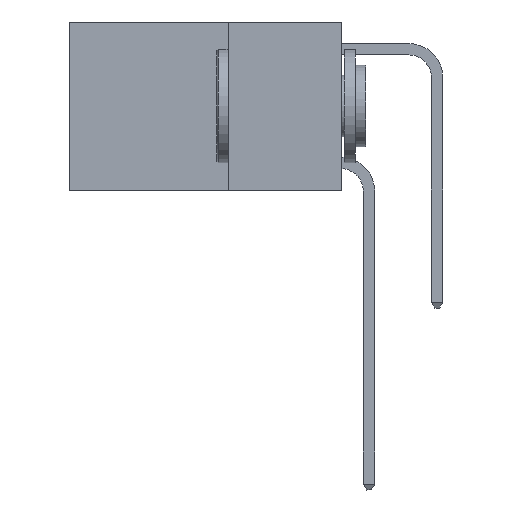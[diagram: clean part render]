
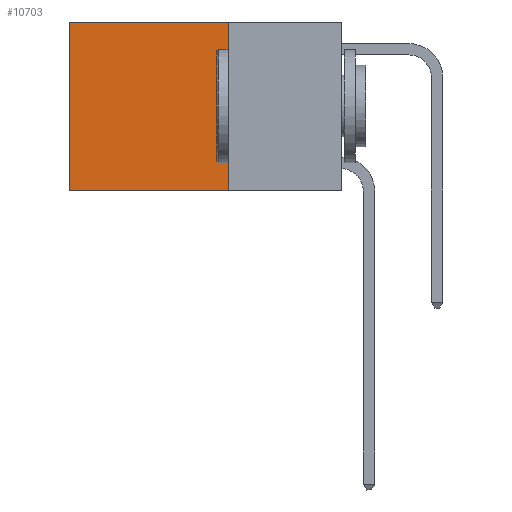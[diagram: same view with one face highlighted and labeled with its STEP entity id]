
A CAD part, left-side view. The second image highlights one B-rep face of the part: STEP entity #10703.
In plain terms, the highlighted planar face has unit normal (-1, 0, 0).
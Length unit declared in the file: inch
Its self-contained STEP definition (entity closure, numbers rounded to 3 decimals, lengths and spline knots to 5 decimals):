
#4 = CARTESIAN_POINT ( 'NONE',  ( 0.2625, 0.6, -0.37 ) ) ;
#459 = DIRECTION ( 'NONE',  ( 0., 0., -1. ) ) ;
#621 = VERTEX_POINT ( 'NONE', #10301 ) ;
#945 = VERTEX_POINT ( 'NONE', #8903 ) ;
#1092 = CARTESIAN_POINT ( 'NONE',  ( 0.2625, 0.6, 0. ) ) ;
#2034 = DIRECTION ( 'NONE',  ( 0., 0., -1. ) ) ;
#2357 = VECTOR ( 'NONE', #9716, 39.37008 ) ;
#2631 = EDGE_LOOP ( 'NONE', ( #8540, #8616, #8750, #8763 ) ) ;
#2666 = DIRECTION ( 'NONE',  ( 1., 0., 0. ) ) ;
#2970 = LINE ( 'NONE', #1092, #4953 ) ;
#3704 = EDGE_CURVE ( 'NONE', #621, #945, #8462, .T. ) ;
#3901 = VECTOR ( 'NONE', #4842, 39.37008 ) ;
#3992 = CARTESIAN_POINT ( 'NONE',  ( 0.2625, 0.25, -0.37 ) ) ;
#4842 = DIRECTION ( 'NONE',  ( 0., 1., 0. ) ) ;
#4857 = VERTEX_POINT ( 'NONE', #4 ) ;
#4953 = VECTOR ( 'NONE', #2034, 39.37008 ) ;
#5801 = LINE ( 'NONE', #3992, #3901 ) ;
#5858 = CARTESIAN_POINT ( 'NONE',  ( 0.2625, 0.25, -0.37 ) ) ;
#5932 = EDGE_CURVE ( 'NONE', #621, #9746, #9826, .T. ) ;
#5971 = PLANE ( 'NONE',  #10980 ) ;
#6028 = FACE_OUTER_BOUND ( 'NONE', #2631, .T. ) ;
#7634 = CARTESIAN_POINT ( 'NONE',  ( 0.2625, 0.25, 0. ) ) ;
#7662 = VECTOR ( 'NONE', #459, 39.37008 ) ;
#8437 = DIRECTION ( 'NONE',  ( 0., 0., -1. ) ) ;
#8462 = LINE ( 'NONE', #8914, #2357 ) ;
#8540 = ORIENTED_EDGE ( 'NONE', *, *, #8690, .T. ) ;
#8616 = ORIENTED_EDGE ( 'NONE', *, *, #8855, .F. ) ;
#8690 = EDGE_CURVE ( 'NONE', #945, #4857, #2970, .T. ) ;
#8750 = ORIENTED_EDGE ( 'NONE', *, *, #5932, .F. ) ;
#8763 = ORIENTED_EDGE ( 'NONE', *, *, #3704, .T. ) ;
#8855 = EDGE_CURVE ( 'NONE', #9746, #4857, #5801, .T. ) ;
#8903 = CARTESIAN_POINT ( 'NONE',  ( 0.2625, 0.6, 0. ) ) ;
#8914 = CARTESIAN_POINT ( 'NONE',  ( 0.2625, 0.25, 0. ) ) ;
#8990 = CARTESIAN_POINT ( 'NONE',  ( 0.2625, 0.25, 0. ) ) ;
#9716 = DIRECTION ( 'NONE',  ( 0., 1., 0. ) ) ;
#9746 = VERTEX_POINT ( 'NONE', #5858 ) ;
#9826 = LINE ( 'NONE', #8990, #7662 ) ;
#10301 = CARTESIAN_POINT ( 'NONE',  ( 0.2625, 0.25, 0. ) ) ;
#10703 = ADVANCED_FACE ( 'NONE', ( #6028 ), #5971, .F. ) ;
#10980 = AXIS2_PLACEMENT_3D ( 'NONE', #7634, #2666, #8437 ) ;
